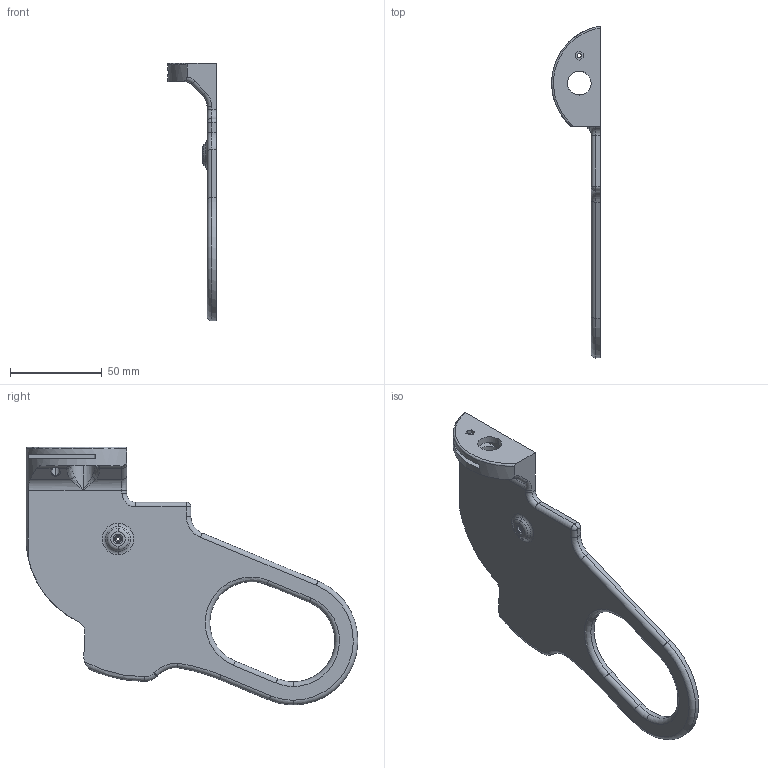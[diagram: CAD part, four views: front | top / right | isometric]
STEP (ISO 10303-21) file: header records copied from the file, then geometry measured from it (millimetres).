
FILE_DESCRIPTION (( 'STEP AP214' ), '1' );
FILE_NAME ('Side_Right.STEP', '2013-11-21T02:42:52', ( '' ), ( '' ), 'SwSTEP 2.0', 'SolidWorks 2013', '' );
FILE_SCHEMA (( 'AUTOMOTIVE_DESIGN' ));
Length unit declared in the file: millimetre
Products named in the file (1): Side_Right
Bounding box: 26.49 x 180.52 x 140.27 mm (x, y, z)
Volume: 67784.6 mm3; surface area: 31444.9 mm2
Topology: 1 solids, 1 shells, 152 faces, 509 edges, 322 vertices
Faces by surface type: cylinder 45, sphere 37, plane 34, torus 26, bspline 8, cone 2
Entity records: 5122 total; most frequent: CARTESIAN_POINT 1385, DIRECTION 832, ORIENTED_EDGE 724, EDGE_CURVE 362, AXIS2_PLACEMENT_3D 355, VERTEX_POINT 250, CIRCLE 210, EDGE_LOOP 202
